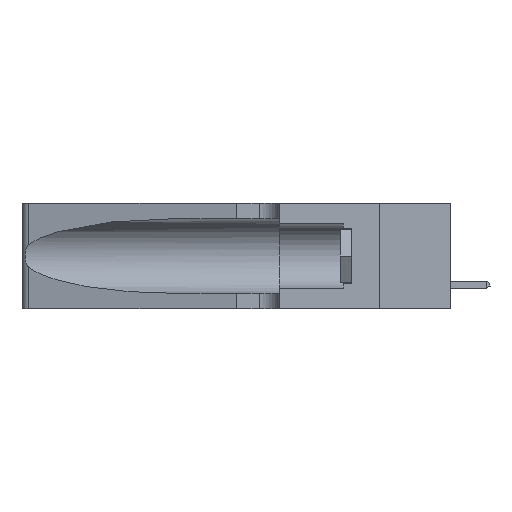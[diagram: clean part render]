
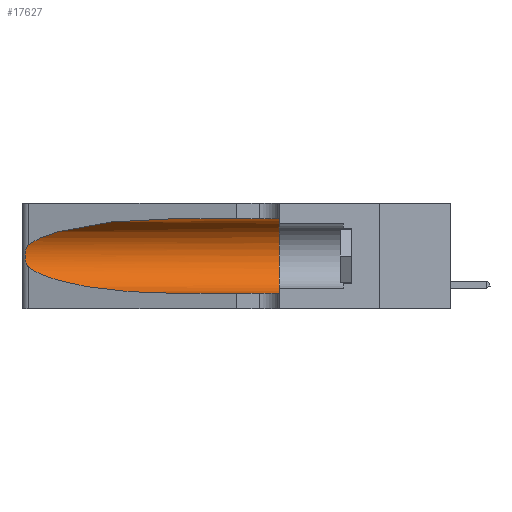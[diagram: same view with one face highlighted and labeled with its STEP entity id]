
A CAD part, left-side view. The second image highlights one B-rep face of the part: STEP entity #17627.
In plain terms, the highlighted cylindrical face has radius 3.308 mm (diameter 6.617 mm), a partial arc.
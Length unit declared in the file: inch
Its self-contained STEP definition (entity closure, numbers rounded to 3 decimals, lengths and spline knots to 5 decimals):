
#483 = VERTEX_POINT ( 'NONE', #23074 ) ;
#1015 = DIRECTION ( 'NONE',  ( 0., 1., 0. ) ) ;
#1016 = ORIENTED_EDGE ( 'NONE', *, *, #13330, .F. ) ;
#4661 = ORIENTED_EDGE ( 'NONE', *, *, #21652, .T. ) ;
#4722 = CYLINDRICAL_SURFACE ( 'NONE', #6502, 0.13025 ) ;
#4763 = CARTESIAN_POINT ( 'NONE',  ( 0.1305, 0.35, 0.185 ) ) ;
#4911 = CARTESIAN_POINT ( 'NONE',  ( 0.26075, 1.23896, 0.178 ) ) ;
#5029 = DIRECTION ( 'NONE',  ( 0., 0., 1. ) ) ;
#5067 = DIRECTION ( 'NONE',  ( 0., -1., 0. ) ) ;
#5917 = VERTEX_POINT ( 'NONE', #22635 ) ;
#6369 = CARTESIAN_POINT ( 'NONE',  ( 0.25487, 1.22718, 0.14631 ) ) ;
#6502 = AXIS2_PLACEMENT_3D ( 'NONE', #18140, #12201, #26393 ) ;
#6555 = CARTESIAN_POINT ( 'NONE',  ( 0.1305, 0.35, 0.05475 ) ) ;
#7274 = DIRECTION ( 'NONE',  ( 0., -1., 0. ) ) ;
#7880 = CARTESIAN_POINT ( 'NONE',  ( 0.2373, 1.15595, 0.28018 ) ) ;
#7958 = EDGE_CURVE ( 'NONE', #8343, #22745, #12375, .T. ) ;
#8262 = CARTESIAN_POINT ( 'NONE',  ( 0.1305, 0.72297, 0.05475 ) ) ;
#8343 = VERTEX_POINT ( 'NONE', #22192 ) ;
#8962 = CARTESIAN_POINT ( 'NONE',  ( 0.25854, 1.2359, 0.20912 ) ) ;
#9032 = EDGE_CURVE ( 'NONE', #483, #11052, #19967, .T. ) ;
#9572 = FACE_OUTER_BOUND ( 'NONE', #17898, .T. ) ;
#10180 = B_SPLINE_CURVE_WITH_KNOTS ( 'NONE', 3,
 ( #17109, #15181, #15258, #20993, #8962, #21071, #15003, #4911, #23181, #23013, #19302, #13007, #25198, #23257 ),
 .UNSPECIFIED., .F., .F.,
 ( 4, 2, 2, 2, 2, 2, 4 ),
 ( 0., 0.00027, 0.00053, 0.00107, 0.0016, 0.00187, 0.00214 ),
 .UNSPECIFIED. ) ;
#10217 = CARTESIAN_POINT ( 'NONE',  ( 0.25487, 1.22718, 0.22369 ) ) ;
#11052 = VERTEX_POINT ( 'NONE', #15848 ) ;
#11061 = CARTESIAN_POINT ( 'NONE',  ( 0.1305, 0.72297, 0.05475 ) ) ;
#11743 = EDGE_CURVE ( 'NONE', #25979, #22745, #20143, .T. ) ;
#12201 = DIRECTION ( 'NONE',  ( 0., -1., 0. ) ) ;
#12375 = CIRCLE ( 'NONE', #23046, 0.13025 ) ;
#12891 = ORIENTED_EDGE ( 'NONE', *, *, #24086, .T. ) ;
#13007 = CARTESIAN_POINT ( 'NONE',  ( 0.25639, 1.23186, 0.15144 ) ) ;
#13228 = CARTESIAN_POINT ( 'NONE',  ( 0.1305, 1.61858, 0.31525 ) ) ;
#13330 = EDGE_CURVE ( 'NONE', #483, #8343, #18816, .T. ) ;
#13797 = VECTOR ( 'NONE', #7274, 39.37008 ) ;
#15003 = CARTESIAN_POINT ( 'NONE',  ( 0.26075, 1.23896, 0.19203 ) ) ;
#15181 = CARTESIAN_POINT ( 'NONE',  ( 0.25555, 1.22994, 0.2215 ) ) ;
#15258 = CARTESIAN_POINT ( 'NONE',  ( 0.25639, 1.23184, 0.21858 ) ) ;
#15330 = ORIENTED_EDGE ( 'NONE', *, *, #11743, .T. ) ;
#15469 = CARTESIAN_POINT ( 'NONE',  ( 0.1305, 1.61858, 0.05475 ) ) ;
#15848 = CARTESIAN_POINT ( 'NONE',  ( 0.25487, 1.22718, 0.22369 ) ) ;
#16387 = CARTESIAN_POINT ( 'NONE',  ( 0.18966, 0.96281, 0.05475 ) ) ;
#16458 =( BOUNDED_CURVE ( )  B_SPLINE_CURVE ( 3, ( #6369, #20458, #16387, #8262 ),
 .UNSPECIFIED., .F., .T. ) 
 B_SPLINE_CURVE_WITH_KNOTS ( ( 4, 4 ),
 ( 3.44316, 4.71239 ),
 .UNSPECIFIED. ) 
 CURVE ( )  GEOMETRIC_REPRESENTATION_ITEM ( )  RATIONAL_B_SPLINE_CURVE ( ( 1., 0.87, 0.87, 1. ) ) 
 REPRESENTATION_ITEM ( '' )  );
#17109 = CARTESIAN_POINT ( 'NONE',  ( 0.25487, 1.22718, 0.22369 ) ) ;
#17627 = ADVANCED_FACE ( 'NONE', ( #9572 ), #4722, .F. ) ;
#17898 = EDGE_LOOP ( 'NONE', ( #20231, #4661, #12891, #15330, #20421, #1016 ) ) ;
#18140 = CARTESIAN_POINT ( 'NONE',  ( 0.1305, 1.61858, 0.185 ) ) ;
#18816 = LINE ( 'NONE', #13228, #22302 ) ;
#19302 = CARTESIAN_POINT ( 'NONE',  ( 0.25789, 1.23486, 0.15765 ) ) ;
#19967 =( BOUNDED_CURVE ( )  B_SPLINE_CURVE ( 3, ( #20357, #20081, #7880, #10217 ),
 .UNSPECIFIED., .F., .F. ) 
 B_SPLINE_CURVE_WITH_KNOTS ( ( 4, 4 ),
 ( 1.5708, 2.84003 ),
 .UNSPECIFIED. ) 
 CURVE ( )  GEOMETRIC_REPRESENTATION_ITEM ( )  RATIONAL_B_SPLINE_CURVE ( ( 1., 0.87, 0.87, 1. ) ) 
 REPRESENTATION_ITEM ( '' )  );
#20081 = CARTESIAN_POINT ( 'NONE',  ( 0.18966, 0.96281, 0.31525 ) ) ;
#20143 = LINE ( 'NONE', #15469, #13797 ) ;
#20231 = ORIENTED_EDGE ( 'NONE', *, *, #9032, .T. ) ;
#20357 = CARTESIAN_POINT ( 'NONE',  ( 0.1305, 0.72297, 0.31525 ) ) ;
#20421 = ORIENTED_EDGE ( 'NONE', *, *, #7958, .F. ) ;
#20458 = CARTESIAN_POINT ( 'NONE',  ( 0.2373, 1.15595, 0.08982 ) ) ;
#20993 = CARTESIAN_POINT ( 'NONE',  ( 0.25787, 1.23484, 0.2124 ) ) ;
#21071 = CARTESIAN_POINT ( 'NONE',  ( 0.26018, 1.23835, 0.19895 ) ) ;
#21652 = EDGE_CURVE ( 'NONE', #11052, #5917, #10180, .T. ) ;
#22192 = CARTESIAN_POINT ( 'NONE',  ( 0.1305, 0.35, 0.31525 ) ) ;
#22302 = VECTOR ( 'NONE', #5067, 39.37008 ) ;
#22635 = CARTESIAN_POINT ( 'NONE',  ( 0.25487, 1.22718, 0.14631 ) ) ;
#22745 = VERTEX_POINT ( 'NONE', #6555 ) ;
#23013 = CARTESIAN_POINT ( 'NONE',  ( 0.25856, 1.23593, 0.16098 ) ) ;
#23046 = AXIS2_PLACEMENT_3D ( 'NONE', #4763, #1015, #5029 ) ;
#23074 = CARTESIAN_POINT ( 'NONE',  ( 0.1305, 0.72297, 0.31525 ) ) ;
#23181 = CARTESIAN_POINT ( 'NONE',  ( 0.26017, 1.23833, 0.17102 ) ) ;
#23257 = CARTESIAN_POINT ( 'NONE',  ( 0.25487, 1.22718, 0.14631 ) ) ;
#24086 = EDGE_CURVE ( 'NONE', #5917, #25979, #16458, .T. ) ;
#25198 = CARTESIAN_POINT ( 'NONE',  ( 0.25555, 1.22993, 0.14849 ) ) ;
#25979 = VERTEX_POINT ( 'NONE', #11061 ) ;
#26393 = DIRECTION ( 'NONE',  ( 0., 0., -1. ) ) ;
